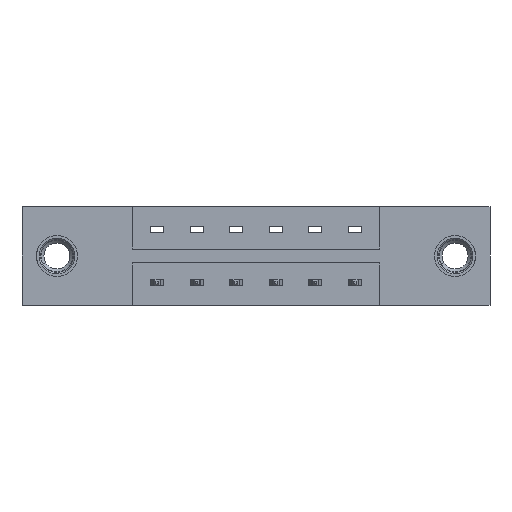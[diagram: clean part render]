
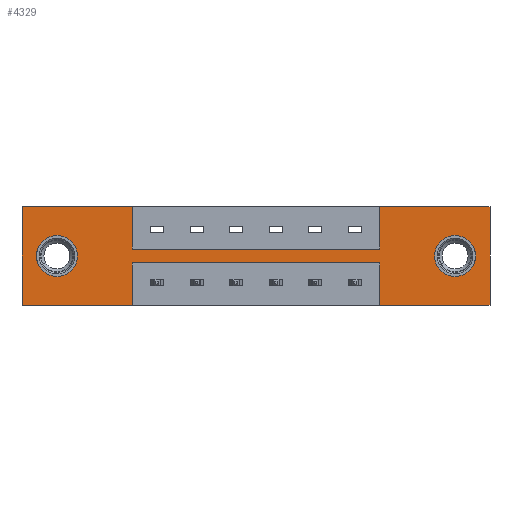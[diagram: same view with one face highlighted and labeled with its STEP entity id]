
A CAD part, front view. The second image highlights one B-rep face of the part: STEP entity #4329.
In plain terms, the highlighted planar face has unit normal (0, -1, 0).
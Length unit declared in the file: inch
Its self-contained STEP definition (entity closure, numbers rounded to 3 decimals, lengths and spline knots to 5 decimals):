
#24 = FACE_BOUND ( 'NONE', #558, .T. ) ;
#53 = EDGE_CURVE ( 'NONE', #8208, #1997, #4375, .T. ) ;
#140 = DIRECTION ( 'NONE',  ( 0., 1., 0. ) ) ;
#150 = LINE ( 'NONE', #8745, #1986 ) ;
#161 = EDGE_CURVE ( 'NONE', #5454, #3681, #4831, .T. ) ;
#282 = ORIENTED_EDGE ( 'NONE', *, *, #53, .T. ) ;
#301 = EDGE_CURVE ( 'NONE', #3681, #7821, #4133, .T. ) ;
#408 = DIRECTION ( 'NONE',  ( 0., 0., 1. ) ) ;
#447 = AXIS2_PLACEMENT_3D ( 'NONE', #7543, #962, #5303 ) ;
#555 = DIRECTION ( 'NONE',  ( 0., 0., 1. ) ) ;
#558 = EDGE_LOOP ( 'NONE', ( #4205, #4621 ) ) ;
#780 = EDGE_CURVE ( 'NONE', #7821, #1964, #7939, .T. ) ;
#821 = CARTESIAN_POINT ( 'NONE',  ( 1.6425, 0., -0.1095 ) ) ;
#962 = DIRECTION ( 'NONE',  ( 0., 1., 0. ) ) ;
#988 = EDGE_LOOP ( 'NONE', ( #3757, #9206, #4492, #5498, #8057, #1848, #6989, #4798, #2746, #4404, #4207, #7121 ) ) ;
#1027 = DIRECTION ( 'NONE',  ( 0., 0., 1. ) ) ;
#1088 = EDGE_CURVE ( 'NONE', #8841, #4301, #6894, .T. ) ;
#1100 = CARTESIAN_POINT ( 'NONE',  ( 0.4175, 0., -0.161 ) ) ;
#1147 = LINE ( 'NONE', #3965, #2977 ) ;
#1225 = LINE ( 'NONE', #5260, #7486 ) ;
#1591 = EDGE_CURVE ( 'NONE', #3704, #3094, #1225, .T. ) ;
#1773 = CARTESIAN_POINT ( 'NONE',  ( 0.4175, 0., -0.214 ) ) ;
#1848 = ORIENTED_EDGE ( 'NONE', *, *, #7980, .F. ) ;
#1874 = VECTOR ( 'NONE', #3643, 39.37008 ) ;
#1964 = VERTEX_POINT ( 'NONE', #5533 ) ;
#1986 = VECTOR ( 'NONE', #8066, 39.37008 ) ;
#1997 = VERTEX_POINT ( 'NONE', #3267 ) ;
#2048 = VERTEX_POINT ( 'NONE', #2717 ) ;
#2292 = VERTEX_POINT ( 'NONE', #8828 ) ;
#2514 = CARTESIAN_POINT ( 'NONE',  ( 0.4175, 0., -0.161 ) ) ;
#2531 = AXIS2_PLACEMENT_3D ( 'NONE', #7545, #140, #5305 ) ;
#2543 = CARTESIAN_POINT ( 'NONE',  ( 1.3575, 0., -0.214 ) ) ;
#2709 = CARTESIAN_POINT ( 'NONE',  ( 0.4175, 0., -0.214 ) ) ;
#2717 = CARTESIAN_POINT ( 'NONE',  ( 0.4175, 0., 0. ) ) ;
#2746 = ORIENTED_EDGE ( 'NONE', *, *, #2944, .F. ) ;
#2805 = EDGE_CURVE ( 'NONE', #4301, #8841, #3864, .T. ) ;
#2826 = CARTESIAN_POINT ( 'NONE',  ( 0., 0., -0.375 ) ) ;
#2838 = ORIENTED_EDGE ( 'NONE', *, *, #6705, .T. ) ;
#2944 = EDGE_CURVE ( 'NONE', #5802, #2292, #3385, .T. ) ;
#2977 = VECTOR ( 'NONE', #7570, 39.37008 ) ;
#3022 = DIRECTION ( 'NONE',  ( 1., 0., 0. ) ) ;
#3094 = VERTEX_POINT ( 'NONE', #8820 ) ;
#3174 = DIRECTION ( 'NONE',  ( -1., 0., 0. ) ) ;
#3194 = CARTESIAN_POINT ( 'NONE',  ( 1.775, 0., 0. ) ) ;
#3267 = CARTESIAN_POINT ( 'NONE',  ( 0.1325, 0., -0.2655 ) ) ;
#3368 = LINE ( 'NONE', #8994, #6858 ) ;
#3385 = LINE ( 'NONE', #5751, #6078 ) ;
#3405 = DIRECTION ( 'NONE',  ( 0., 0., -1. ) ) ;
#3412 = EDGE_CURVE ( 'NONE', #2048, #9379, #3619, .T. ) ;
#3443 = DIRECTION ( 'NONE',  ( 0., 0., -1. ) ) ;
#3452 = DIRECTION ( 'NONE',  ( 0., 1., 0. ) ) ;
#3553 = EDGE_CURVE ( 'NONE', #1964, #5802, #6292, .T. ) ;
#3554 = AXIS2_PLACEMENT_3D ( 'NONE', #6198, #9110, #4707 ) ;
#3600 = FACE_BOUND ( 'NONE', #5915, .T. ) ;
#3619 = LINE ( 'NONE', #1100, #4091 ) ;
#3643 = DIRECTION ( 'NONE',  ( -1., 0., 0. ) ) ;
#3681 = VERTEX_POINT ( 'NONE', #3931 ) ;
#3704 = VERTEX_POINT ( 'NONE', #5302 ) ;
#3705 = CARTESIAN_POINT ( 'NONE',  ( 1.6425, 0., -0.2655 ) ) ;
#3741 = EDGE_CURVE ( 'NONE', #8789, #5454, #3368, .T. ) ;
#3757 = ORIENTED_EDGE ( 'NONE', *, *, #161, .F. ) ;
#3864 = CIRCLE ( 'NONE', #7523, 0.078 ) ;
#3931 = CARTESIAN_POINT ( 'NONE',  ( 1.3575, 0., -0.214 ) ) ;
#3955 = CARTESIAN_POINT ( 'NONE',  ( 0.4175, 0., -0.214 ) ) ;
#3965 = CARTESIAN_POINT ( 'NONE',  ( 0., 0., 0. ) ) ;
#4091 = VECTOR ( 'NONE', #3405, 39.37008 ) ;
#4129 = EDGE_CURVE ( 'NONE', #7874, #8789, #150, .T. ) ;
#4133 = LINE ( 'NONE', #1773, #5887 ) ;
#4205 = ORIENTED_EDGE ( 'NONE', *, *, #2805, .T. ) ;
#4207 = ORIENTED_EDGE ( 'NONE', *, *, #780, .F. ) ;
#4301 = VERTEX_POINT ( 'NONE', #821 ) ;
#4329 = ADVANCED_FACE ( 'NONE', ( #24, #3600, #7665 ), #6840, .T. ) ;
#4375 = CIRCLE ( 'NONE', #2531, 0.078 ) ;
#4404 = ORIENTED_EDGE ( 'NONE', *, *, #3553, .F. ) ;
#4492 = ORIENTED_EDGE ( 'NONE', *, *, #4129, .F. ) ;
#4496 = CARTESIAN_POINT ( 'NONE',  ( 0., 0., 0. ) ) ;
#4621 = ORIENTED_EDGE ( 'NONE', *, *, #1088, .T. ) ;
#4707 = DIRECTION ( 'NONE',  ( 0., 0., -1. ) ) ;
#4798 = ORIENTED_EDGE ( 'NONE', *, *, #4929, .F. ) ;
#4831 = LINE ( 'NONE', #2543, #5542 ) ;
#4929 = EDGE_CURVE ( 'NONE', #2292, #2048, #1147, .T. ) ;
#5260 = CARTESIAN_POINT ( 'NONE',  ( 1.3575, 0., -0.161 ) ) ;
#5302 = CARTESIAN_POINT ( 'NONE',  ( 1.3575, 0., -0.161 ) ) ;
#5303 = DIRECTION ( 'NONE',  ( 0., 0., -1. ) ) ;
#5305 = DIRECTION ( 'NONE',  ( 0., 0., 1. ) ) ;
#5328 = VECTOR ( 'NONE', #3022, 39.37008 ) ;
#5454 = VERTEX_POINT ( 'NONE', #9169 ) ;
#5498 = ORIENTED_EDGE ( 'NONE', *, *, #7247, .F. ) ;
#5533 = CARTESIAN_POINT ( 'NONE',  ( 0.4175, 0., -0.375 ) ) ;
#5542 = VECTOR ( 'NONE', #1027, 39.37008 ) ;
#5647 = VECTOR ( 'NONE', #3443, 39.37008 ) ;
#5751 = CARTESIAN_POINT ( 'NONE',  ( 0., 0., 0. ) ) ;
#5796 = LINE ( 'NONE', #8026, #7290 ) ;
#5802 = VERTEX_POINT ( 'NONE', #9387 ) ;
#5808 = LINE ( 'NONE', #4496, #5328 ) ;
#5887 = VECTOR ( 'NONE', #3174, 39.37008 ) ;
#5915 = EDGE_LOOP ( 'NONE', ( #282, #2838 ) ) ;
#6078 = VECTOR ( 'NONE', #555, 39.37008 ) ;
#6198 = CARTESIAN_POINT ( 'NONE',  ( 0., 0., -0.375 ) ) ;
#6292 = LINE ( 'NONE', #2826, #1874 ) ;
#6424 = DIRECTION ( 'NONE',  ( 0., 0., -1. ) ) ;
#6705 = EDGE_CURVE ( 'NONE', #1997, #8208, #7322, .T. ) ;
#6748 = DIRECTION ( 'NONE',  ( 0., 0., 1. ) ) ;
#6840 = PLANE ( 'NONE',  #3554 ) ;
#6858 = VECTOR ( 'NONE', #9024, 39.37008 ) ;
#6894 = CIRCLE ( 'NONE', #447, 0.078 ) ;
#6979 = DIRECTION ( 'NONE',  ( 0., 1., 0. ) ) ;
#6989 = ORIENTED_EDGE ( 'NONE', *, *, #3412, .F. ) ;
#7121 = ORIENTED_EDGE ( 'NONE', *, *, #301, .F. ) ;
#7247 = EDGE_CURVE ( 'NONE', #3094, #7874, #5808, .T. ) ;
#7290 = VECTOR ( 'NONE', #9451, 39.37008 ) ;
#7302 = AXIS2_PLACEMENT_3D ( 'NONE', #7723, #6979, #408 ) ;
#7322 = CIRCLE ( 'NONE', #7302, 0.078 ) ;
#7486 = VECTOR ( 'NONE', #6748, 39.37008 ) ;
#7523 = AXIS2_PLACEMENT_3D ( 'NONE', #7870, #3452, #6424 ) ;
#7543 = CARTESIAN_POINT ( 'NONE',  ( 1.6425, 0., -0.1875 ) ) ;
#7545 = CARTESIAN_POINT ( 'NONE',  ( 0.1325, 0., -0.1875 ) ) ;
#7570 = DIRECTION ( 'NONE',  ( 1., 0., 0. ) ) ;
#7614 = CARTESIAN_POINT ( 'NONE',  ( 0.1325, 0., -0.1095 ) ) ;
#7665 = FACE_OUTER_BOUND ( 'NONE', #988, .T. ) ;
#7723 = CARTESIAN_POINT ( 'NONE',  ( 0.1325, 0., -0.1875 ) ) ;
#7821 = VERTEX_POINT ( 'NONE', #3955 ) ;
#7870 = CARTESIAN_POINT ( 'NONE',  ( 1.6425, 0., -0.1875 ) ) ;
#7874 = VERTEX_POINT ( 'NONE', #3194 ) ;
#7939 = LINE ( 'NONE', #2709, #5647 ) ;
#7980 = EDGE_CURVE ( 'NONE', #9379, #3704, #5796, .T. ) ;
#8026 = CARTESIAN_POINT ( 'NONE',  ( 0.4175, 0., -0.161 ) ) ;
#8057 = ORIENTED_EDGE ( 'NONE', *, *, #1591, .F. ) ;
#8066 = DIRECTION ( 'NONE',  ( 0., 0., -1. ) ) ;
#8208 = VERTEX_POINT ( 'NONE', #7614 ) ;
#8745 = CARTESIAN_POINT ( 'NONE',  ( 1.775, 0., 0. ) ) ;
#8789 = VERTEX_POINT ( 'NONE', #8932 ) ;
#8820 = CARTESIAN_POINT ( 'NONE',  ( 1.3575, 0., 0. ) ) ;
#8828 = CARTESIAN_POINT ( 'NONE',  ( 0., 0., 0. ) ) ;
#8841 = VERTEX_POINT ( 'NONE', #3705 ) ;
#8932 = CARTESIAN_POINT ( 'NONE',  ( 1.775, 0., -0.375 ) ) ;
#8994 = CARTESIAN_POINT ( 'NONE',  ( 0., 0., -0.375 ) ) ;
#9024 = DIRECTION ( 'NONE',  ( -1., 0., 0. ) ) ;
#9110 = DIRECTION ( 'NONE',  ( 0., -1., 0. ) ) ;
#9169 = CARTESIAN_POINT ( 'NONE',  ( 1.3575, 0., -0.375 ) ) ;
#9206 = ORIENTED_EDGE ( 'NONE', *, *, #3741, .F. ) ;
#9379 = VERTEX_POINT ( 'NONE', #2514 ) ;
#9387 = CARTESIAN_POINT ( 'NONE',  ( 0., 0., -0.375 ) ) ;
#9451 = DIRECTION ( 'NONE',  ( 1., 0., 0. ) ) ;
